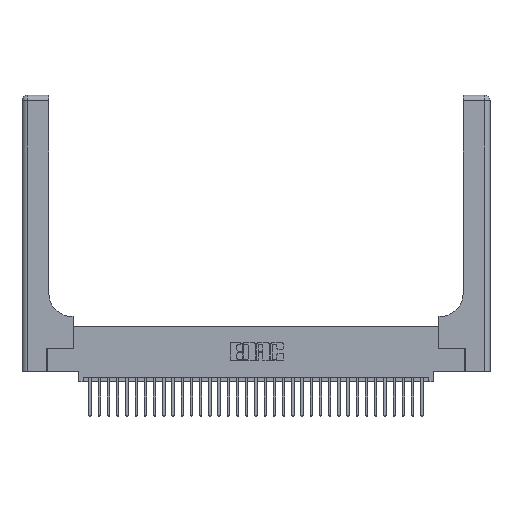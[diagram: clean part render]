
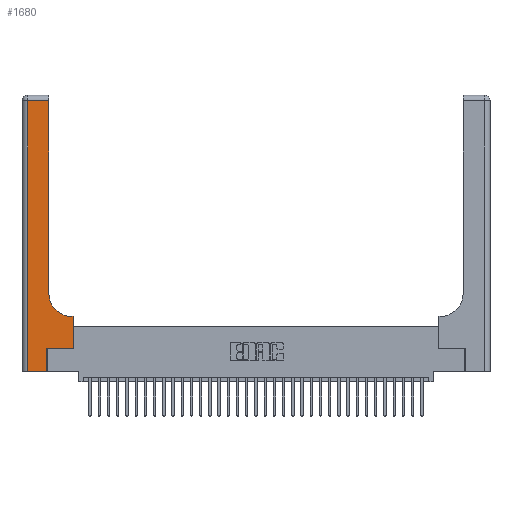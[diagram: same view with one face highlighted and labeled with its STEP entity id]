
A CAD part, top view. The second image highlights one B-rep face of the part: STEP entity #1680.
In plain terms, the highlighted planar face has unit normal (0, 0, 1).
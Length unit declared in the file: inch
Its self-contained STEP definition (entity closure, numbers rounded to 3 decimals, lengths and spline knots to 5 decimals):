
#161 = VERTEX_POINT ( 'NONE', #17791 ) ;
#605 = VERTEX_POINT ( 'NONE', #14134 ) ;
#619 = VECTOR ( 'NONE', #30059, 39.37008 ) ;
#1623 = ORIENTED_EDGE ( 'NONE', *, *, #5378, .T. ) ;
#1657 = VERTEX_POINT ( 'NONE', #26926 ) ;
#1680 = ADVANCED_FACE ( 'NONE', ( #29969 ), #13600, .F. ) ;
#4010 = DIRECTION ( 'NONE',  ( 0., 1., 0. ) ) ;
#4098 = ORIENTED_EDGE ( 'NONE', *, *, #16179, .T. ) ;
#4687 = LINE ( 'NONE', #13110, #19274 ) ;
#5331 = CARTESIAN_POINT ( 'NONE',  ( 0., 3., 0.37 ) ) ;
#5378 = EDGE_CURVE ( 'NONE', #16388, #1657, #7904, .T. ) ;
#5655 = AXIS2_PLACEMENT_3D ( 'NONE', #5331, #8235, #27152 ) ;
#7361 = EDGE_CURVE ( 'NONE', #23215, #161, #33489, .T. ) ;
#7517 = LINE ( 'NONE', #18183, #21175 ) ;
#7604 = CARTESIAN_POINT ( 'NONE',  ( 0.2915, 0.85, 0.37 ) ) ;
#7833 = DIRECTION ( 'NONE',  ( 0., -1., 0. ) ) ;
#7904 = LINE ( 'NONE', #19486, #28623 ) ;
#7967 = CARTESIAN_POINT ( 'NONE',  ( 0.2915, 2.94, 0.37 ) ) ;
#8235 = DIRECTION ( 'NONE',  ( 0., 0., -1. ) ) ;
#8815 = VECTOR ( 'NONE', #4010, 39.37008 ) ;
#8842 = EDGE_LOOP ( 'NONE', ( #28153, #25204, #20140, #28829, #16597, #1623, #4098, #25873, #34780 ) ) ;
#10496 = VERTEX_POINT ( 'NONE', #26299 ) ;
#11255 = VECTOR ( 'NONE', #17012, 39.37008 ) ;
#12690 = VERTEX_POINT ( 'NONE', #7604 ) ;
#12741 = EDGE_CURVE ( 'NONE', #10496, #33787, #13870, .T. ) ;
#13110 = CARTESIAN_POINT ( 'NONE',  ( 0., 2.94, 0.37 ) ) ;
#13489 = VECTOR ( 'NONE', #23756, 39.37008 ) ;
#13600 = PLANE ( 'NONE',  #5655 ) ;
#13870 = LINE ( 'NONE', #16113, #34392 ) ;
#14134 = CARTESIAN_POINT ( 'NONE',  ( 0.269, 0., 0.37 ) ) ;
#14350 = LINE ( 'NONE', #21069, #13489 ) ;
#14385 = DIRECTION ( 'NONE',  ( 0., 0., -1. ) ) ;
#15227 = CIRCLE ( 'NONE', #22006, 0.25 ) ;
#15250 = LINE ( 'NONE', #20396, #8815 ) ;
#16113 = CARTESIAN_POINT ( 'NONE',  ( 0.06, 3., 0.37 ) ) ;
#16139 = LINE ( 'NONE', #16739, #619 ) ;
#16179 = EDGE_CURVE ( 'NONE', #1657, #23215, #7517, .T. ) ;
#16380 = CARTESIAN_POINT ( 'NONE',  ( 0.269, 0.25, 0.37 ) ) ;
#16388 = VERTEX_POINT ( 'NONE', #16380 ) ;
#16597 = ORIENTED_EDGE ( 'NONE', *, *, #31928, .T. ) ;
#16739 = CARTESIAN_POINT ( 'NONE',  ( 0., 0., 0.37 ) ) ;
#16765 = DIRECTION ( 'NONE',  ( 1., 0., 0. ) ) ;
#16869 = VERTEX_POINT ( 'NONE', #7967 ) ;
#17012 = DIRECTION ( 'NONE',  ( -1., 0., 0. ) ) ;
#17791 = CARTESIAN_POINT ( 'NONE',  ( 0.5415, 0.6, 0.37 ) ) ;
#18183 = CARTESIAN_POINT ( 'NONE',  ( 0.5585, 0.25, 0.37 ) ) ;
#19274 = VECTOR ( 'NONE', #34559, 39.37008 ) ;
#19486 = CARTESIAN_POINT ( 'NONE',  ( 0.269, 0.25, 0.37 ) ) ;
#20140 = ORIENTED_EDGE ( 'NONE', *, *, #12741, .T. ) ;
#20396 = CARTESIAN_POINT ( 'NONE',  ( 0.2915, 3., 0.37 ) ) ;
#21069 = CARTESIAN_POINT ( 'NONE',  ( 0.269, 0., 0.37 ) ) ;
#21075 = CARTESIAN_POINT ( 'NONE',  ( 0.06, 0., 0.37 ) ) ;
#21175 = VECTOR ( 'NONE', #26226, 39.37008 ) ;
#22006 = AXIS2_PLACEMENT_3D ( 'NONE', #30478, #14385, #33118 ) ;
#22385 = EDGE_CURVE ( 'NONE', #12690, #16869, #15250, .T. ) ;
#23215 = VERTEX_POINT ( 'NONE', #30429 ) ;
#23601 = EDGE_CURVE ( 'NONE', #16869, #10496, #4687, .T. ) ;
#23756 = DIRECTION ( 'NONE',  ( 0., 1., 0. ) ) ;
#25204 = ORIENTED_EDGE ( 'NONE', *, *, #23601, .T. ) ;
#25686 = EDGE_CURVE ( 'NONE', #33787, #605, #16139, .T. ) ;
#25873 = ORIENTED_EDGE ( 'NONE', *, *, #7361, .T. ) ;
#26132 = EDGE_CURVE ( 'NONE', #161, #12690, #15227, .T. ) ;
#26226 = DIRECTION ( 'NONE',  ( 0., 1., 0. ) ) ;
#26299 = CARTESIAN_POINT ( 'NONE',  ( 0.06, 2.94, 0.37 ) ) ;
#26926 = CARTESIAN_POINT ( 'NONE',  ( 0.5585, 0.25, 0.37 ) ) ;
#27152 = DIRECTION ( 'NONE',  ( -1., 0., 0. ) ) ;
#27643 = CARTESIAN_POINT ( 'NONE',  ( 0.2915, 0.6, 0.37 ) ) ;
#28153 = ORIENTED_EDGE ( 'NONE', *, *, #22385, .T. ) ;
#28623 = VECTOR ( 'NONE', #16765, 39.37008 ) ;
#28829 = ORIENTED_EDGE ( 'NONE', *, *, #25686, .T. ) ;
#29969 = FACE_OUTER_BOUND ( 'NONE', #8842, .T. ) ;
#30059 = DIRECTION ( 'NONE',  ( 1., 0., 0. ) ) ;
#30429 = CARTESIAN_POINT ( 'NONE',  ( 0.5585, 0.6, 0.37 ) ) ;
#30478 = CARTESIAN_POINT ( 'NONE',  ( 0.5415, 0.85, 0.37 ) ) ;
#31928 = EDGE_CURVE ( 'NONE', #605, #16388, #14350, .T. ) ;
#33118 = DIRECTION ( 'NONE',  ( 1., 0., 0. ) ) ;
#33489 = LINE ( 'NONE', #27643, #11255 ) ;
#33787 = VERTEX_POINT ( 'NONE', #21075 ) ;
#34392 = VECTOR ( 'NONE', #7833, 39.37008 ) ;
#34559 = DIRECTION ( 'NONE',  ( -1., 0., 0. ) ) ;
#34780 = ORIENTED_EDGE ( 'NONE', *, *, #26132, .T. ) ;
